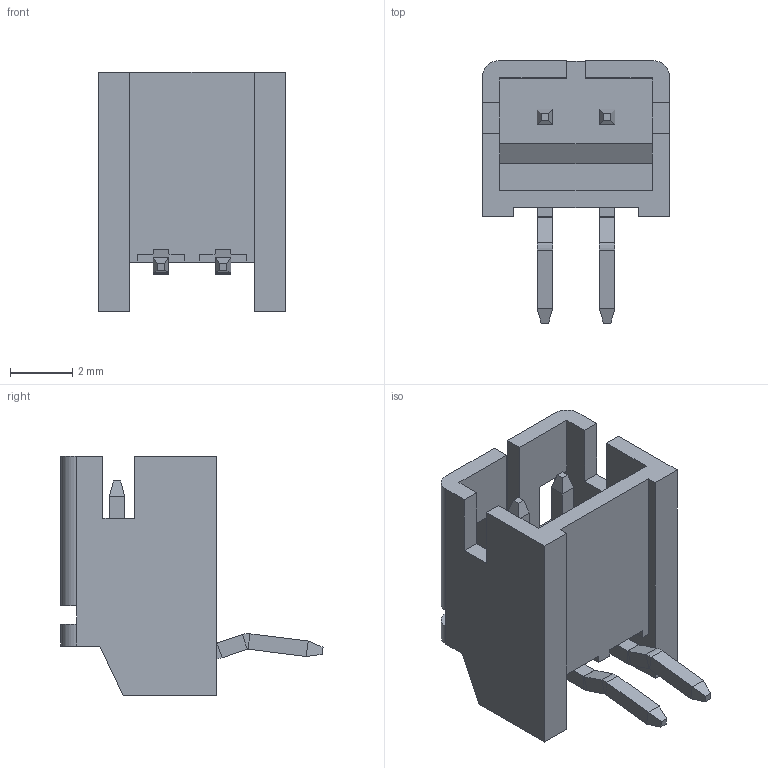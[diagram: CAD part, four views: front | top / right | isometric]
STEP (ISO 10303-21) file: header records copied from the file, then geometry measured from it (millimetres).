
FILE_DESCRIPTION (( 'STEP AP203' ), '1' );
FILE_NAME ('140-502-415-000.STEP', '2020-03-31T19:40:04', ( '' ), ( '' ), 'SwSTEP 2.0', 'SolidWorks 2016', '' );
FILE_SCHEMA (( 'CONFIG_CONTROL_DESIGN' ));
Length unit declared in the file: millimetre
Products named in the file (3): RA Housing_502; 140-502-415-000; RA Contact_Kink
Assembly tree (3 placements, depth 2):
  140-502-415-000
    RA Housing_502
    RA Contact_Kink  x2
Bounding box: 6 x 8.41 x 7.7 mm (x, y, z)
Volume: 98.9 mm3; surface area: 354.1 mm2
Topology: 3 solids, 3 shells, 139 faces, 337 edges, 202 vertices
Faces by surface type: plane 123, cylinder 16
Entity records: 3340 total; most frequent: CARTESIAN_POINT 530, ORIENTED_EDGE 522, DIRECTION 495, EDGE_CURVE 261, VECTOR 241, LINE 241, VERTEX_POINT 162, AXIS2_PLACEMENT_3D 127
